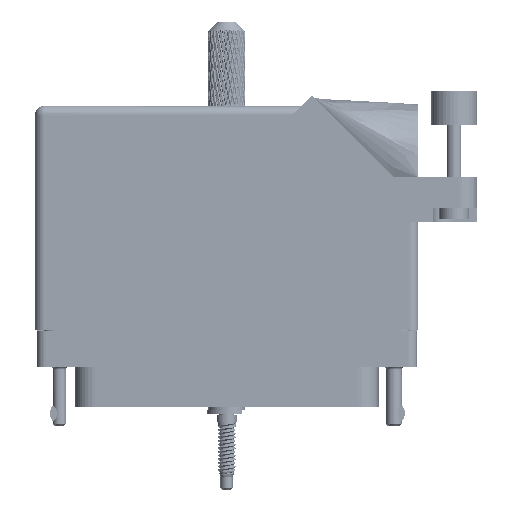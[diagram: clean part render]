
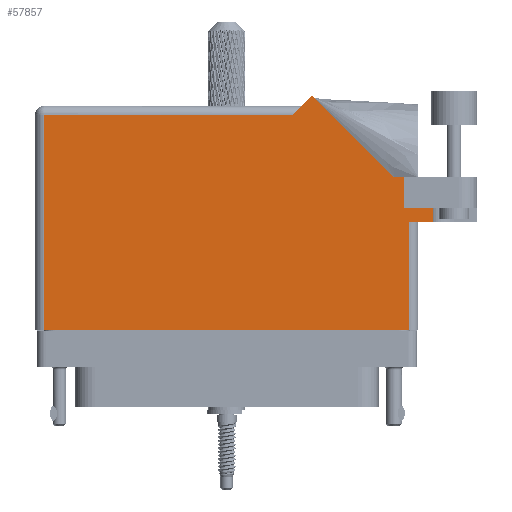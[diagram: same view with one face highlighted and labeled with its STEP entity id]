
A CAD part, front view. The second image highlights one B-rep face of the part: STEP entity #57857.
In plain terms, the highlighted face is planar.
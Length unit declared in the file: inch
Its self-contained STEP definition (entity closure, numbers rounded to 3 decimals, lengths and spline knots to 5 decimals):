
#9 = CARTESIAN_POINT ( 'NONE',  ( -1.306, -0.1, 0.455 ) ) ;
#2141 = CARTESIAN_POINT ( 'NONE',  ( -1.244, -0.1, 0.455 ) ) ;
#3206 = EDGE_CURVE ( 'NONE', #94086, #10417, #112117, .T. ) ;
#4660 = ORIENTED_EDGE ( 'NONE', *, *, #21694, .T. ) ;
#4782 = VECTOR ( 'NONE', #83418, 39.37008 ) ;
#6232 = VERTEX_POINT ( 'NONE', #40348 ) ;
#6892 = ORIENTED_EDGE ( 'NONE', *, *, #3206, .T. ) ;
#9167 = DIRECTION ( 'NONE',  ( 0., 0., -1. ) ) ;
#9441 = ORIENTED_EDGE ( 'NONE', *, *, #81704, .F. ) ;
#9628 = VECTOR ( 'NONE', #111022, 39.37008 ) ;
#9808 = CARTESIAN_POINT ( 'NONE',  ( 1.206, 0.944, 0.455 ) ) ;
#9963 = EDGE_CURVE ( 'NONE', #89355, #6232, #109711, .T. ) ;
#10417 = VERTEX_POINT ( 'NONE', #72887 ) ;
#10834 = LINE ( 'NONE', #21706, #98478 ) ;
#11246 = CARTESIAN_POINT ( 'NONE',  ( -1.244, 1.368, 0.455 ) ) ;
#14127 = LINE ( 'NONE', #122504, #9628 ) ;
#14559 = FACE_OUTER_BOUND ( 'NONE', #119399, .T. ) ;
#14624 = CARTESIAN_POINT ( 'NONE',  ( 1.206, 0.731, 0.455 ) ) ;
#19226 = ORIENTED_EDGE ( 'NONE', *, *, #48493, .F. ) ;
#21694 = EDGE_CURVE ( 'NONE', #6232, #79321, #34903, .T. ) ;
#21706 = CARTESIAN_POINT ( 'NONE',  ( 1.206, 0.731, 0.455 ) ) ;
#23254 = LINE ( 'NONE', #14624, #4782 ) ;
#23822 = VERTEX_POINT ( 'NONE', #112763 ) ;
#29359 = CARTESIAN_POINT ( 'NONE',  ( -1.306, 1.43, 0.455 ) ) ;
#30975 = LINE ( 'NONE', #118769, #126141 ) ;
#31428 = ORIENTED_EDGE ( 'NONE', *, *, #100861, .T. ) ;
#32386 = VECTOR ( 'NONE', #66409, 39.37008 ) ;
#32450 = DIRECTION ( 'NONE',  ( 0., 1., 0. ) ) ;
#34903 = LINE ( 'NONE', #77130, #119352 ) ;
#40348 = CARTESIAN_POINT ( 'NONE',  ( 1.14042, 0.944, 0.455 ) ) ;
#43740 = EDGE_CURVE ( 'NONE', #102655, #94086, #63626, .T. ) ;
#48118 = EDGE_CURVE ( 'NONE', #120032, #90140, #72376, .T. ) ;
#48288 = VECTOR ( 'NONE', #115179, 39.37008 ) ;
#48493 = EDGE_CURVE ( 'NONE', #51319, #90140, #69197, .T. ) ;
#49789 = DIRECTION ( 'NONE',  ( 1., 0., 0. ) ) ;
#51319 = VERTEX_POINT ( 'NONE', #58504 ) ;
#55332 = VECTOR ( 'NONE', #49789, 39.37008 ) ;
#55407 = ORIENTED_EDGE ( 'NONE', *, *, #82380, .T. ) ;
#55961 = VECTOR ( 'NONE', #61844, 39.37008 ) ;
#57857 = ADVANCED_FACE ( 'NONE', ( #14559 ), #116479, .F. ) ;
#58504 = CARTESIAN_POINT ( 'NONE',  ( 1.4075, 0.731, 0.455 ) ) ;
#59272 = AXIS2_PLACEMENT_3D ( 'NONE', #29359, #9167, #87378 ) ;
#61777 = DIRECTION ( 'NONE',  ( 1., 0., 0. ) ) ;
#61844 = DIRECTION ( 'NONE',  ( 0., -1., 0. ) ) ;
#61994 = ORIENTED_EDGE ( 'NONE', *, *, #9963, .T. ) ;
#63604 = EDGE_CURVE ( 'NONE', #79321, #122999, #104192, .T. ) ;
#63626 = LINE ( 'NONE', #2141, #55961 ) ;
#65117 = CARTESIAN_POINT ( 'NONE',  ( 1.4075, 1.06177, 0.455 ) ) ;
#66409 = DIRECTION ( 'NONE',  ( 0., -1., 0. ) ) ;
#67374 = CARTESIAN_POINT ( 'NONE',  ( 0.451, 1.368, 0.455 ) ) ;
#69197 = LINE ( 'NONE', #65117, #32386 ) ;
#72376 = LINE ( 'NONE', #72443, #81666 ) ;
#72443 = CARTESIAN_POINT ( 'NONE',  ( 1.306, 0.637, 0.455 ) ) ;
#72887 = CARTESIAN_POINT ( 'NONE',  ( 1.244, -0.1, 0.455 ) ) ;
#76518 = CARTESIAN_POINT ( 'NONE',  ( 0.513, 1.43, 0.455 ) ) ;
#77130 = CARTESIAN_POINT ( 'NONE',  ( 1.14042, 0.944, 0.455 ) ) ;
#78159 = VECTOR ( 'NONE', #86830, 39.37008 ) ;
#79321 = VERTEX_POINT ( 'NONE', #107716 ) ;
#81666 = VECTOR ( 'NONE', #61777, 39.37008 ) ;
#81704 = EDGE_CURVE ( 'NONE', #23822, #51319, #23254, .T. ) ;
#82380 = EDGE_CURVE ( 'NONE', #23822, #89355, #10834, .T. ) ;
#83418 = DIRECTION ( 'NONE',  ( 1., 0., 0. ) ) ;
#86830 = DIRECTION ( 'NONE',  ( -0.707, -0.707, 0. ) ) ;
#87378 = DIRECTION ( 'NONE',  ( -1., 0., 0. ) ) ;
#89355 = VERTEX_POINT ( 'NONE', #9808 ) ;
#89904 = EDGE_CURVE ( 'NONE', #10417, #120032, #30975, .T. ) ;
#90140 = VERTEX_POINT ( 'NONE', #124234 ) ;
#94086 = VERTEX_POINT ( 'NONE', #122071 ) ;
#95578 = DIRECTION ( 'NONE',  ( -0.707, 0.707, 0. ) ) ;
#98478 = VECTOR ( 'NONE', #32450, 39.37008 ) ;
#99513 = DIRECTION ( 'NONE',  ( 0., 1., 0. ) ) ;
#99579 = ORIENTED_EDGE ( 'NONE', *, *, #43740, .T. ) ;
#100861 = EDGE_CURVE ( 'NONE', #122999, #102655, #14127, .T. ) ;
#102655 = VERTEX_POINT ( 'NONE', #11246 ) ;
#104192 = LINE ( 'NONE', #76518, #78159 ) ;
#104799 = CARTESIAN_POINT ( 'NONE',  ( 1.244, 0.637, 0.455 ) ) ;
#105661 = ORIENTED_EDGE ( 'NONE', *, *, #89904, .T. ) ;
#107716 = CARTESIAN_POINT ( 'NONE',  ( 0.58371, 1.50071, 0.455 ) ) ;
#109049 = ORIENTED_EDGE ( 'NONE', *, *, #48118, .T. ) ;
#109711 = LINE ( 'NONE', #125429, #48288 ) ;
#111022 = DIRECTION ( 'NONE',  ( -1., 0., 0. ) ) ;
#112117 = LINE ( 'NONE', #9, #55332 ) ;
#112763 = CARTESIAN_POINT ( 'NONE',  ( 1.206, 0.731, 0.455 ) ) ;
#115179 = DIRECTION ( 'NONE',  ( -1., 0., 0. ) ) ;
#116479 = PLANE ( 'NONE',  #59272 ) ;
#118769 = CARTESIAN_POINT ( 'NONE',  ( 1.244, 0.637, 0.455 ) ) ;
#119352 = VECTOR ( 'NONE', #95578, 39.37008 ) ;
#119399 = EDGE_LOOP ( 'NONE', ( #6892, #105661, #109049, #19226, #9441, #55407, #61994, #4660, #122734, #31428, #99579 ) ) ;
#120032 = VERTEX_POINT ( 'NONE', #104799 ) ;
#122071 = CARTESIAN_POINT ( 'NONE',  ( -1.244, -0.1, 0.455 ) ) ;
#122504 = CARTESIAN_POINT ( 'NONE',  ( -1.306, 1.368, 0.455 ) ) ;
#122734 = ORIENTED_EDGE ( 'NONE', *, *, #63604, .T. ) ;
#122999 = VERTEX_POINT ( 'NONE', #67374 ) ;
#124234 = CARTESIAN_POINT ( 'NONE',  ( 1.4075, 0.637, 0.455 ) ) ;
#125429 = CARTESIAN_POINT ( 'NONE',  ( 1.706, 0.944, 0.455 ) ) ;
#126141 = VECTOR ( 'NONE', #99513, 39.37008 ) ;
